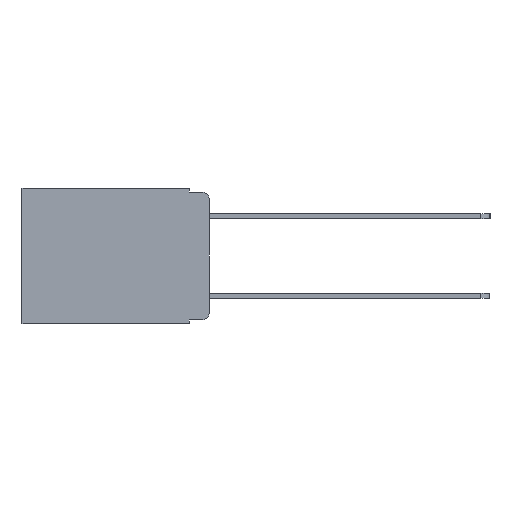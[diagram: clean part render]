
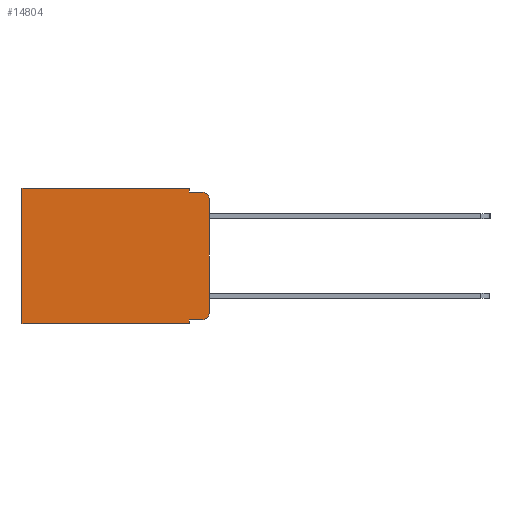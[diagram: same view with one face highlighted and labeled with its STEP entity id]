
A CAD part, left-side view. The second image highlights one B-rep face of the part: STEP entity #14804.
In plain terms, the highlighted planar face has unit normal (-1, 0, 0).
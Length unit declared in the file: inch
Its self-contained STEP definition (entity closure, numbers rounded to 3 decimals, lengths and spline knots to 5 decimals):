
#355 = CARTESIAN_POINT ( 'NONE',  ( 0.298, 0.02, -0.03 ) ) ;
#734 = ORIENTED_EDGE ( 'NONE', *, *, #15490, .T. ) ;
#1044 = DIRECTION ( 'NONE',  ( -1., 0., 0. ) ) ;
#1151 = CARTESIAN_POINT ( 'NONE',  ( 0.298, 0., 0. ) ) ;
#1169 = EDGE_CURVE ( 'NONE', #6300, #10771, #10033, .T. ) ;
#1171 = CARTESIAN_POINT ( 'NONE',  ( 0.298, 0.051, 0. ) ) ;
#1495 = VERTEX_POINT ( 'NONE', #5704 ) ;
#1880 = DIRECTION ( 'NONE',  ( 0., 0., -1. ) ) ;
#1925 = EDGE_LOOP ( 'NONE', ( #15709, #5571, #3028, #11888, #15908, #13172, #9977, #6684, #4193, #734 ) ) ;
#2404 = VECTOR ( 'NONE', #9166, 39.37008 ) ;
#2518 = CARTESIAN_POINT ( 'NONE',  ( 0.298, 0., -0.03 ) ) ;
#2577 = VECTOR ( 'NONE', #15664, 39.37008 ) ;
#2625 = DIRECTION ( 'NONE',  ( 0., 0., -1. ) ) ;
#3028 = ORIENTED_EDGE ( 'NONE', *, *, #18139, .F. ) ;
#3727 = CARTESIAN_POINT ( 'NONE',  ( 0.298, 0., -0.343 ) ) ;
#3985 = CARTESIAN_POINT ( 'NONE',  ( 0.298, 0.051, -0.333 ) ) ;
#4073 = LINE ( 'NONE', #1151, #11562 ) ;
#4193 = ORIENTED_EDGE ( 'NONE', *, *, #10591, .T. ) ;
#4564 = CIRCLE ( 'NONE', #8751, 0.02 ) ;
#4751 = DIRECTION ( 'NONE',  ( 0., -1., 0. ) ) ;
#5084 = VERTEX_POINT ( 'NONE', #9344 ) ;
#5256 = PLANE ( 'NONE',  #6609 ) ;
#5445 = CARTESIAN_POINT ( 'NONE',  ( 0.298, 0.02, -0.333 ) ) ;
#5571 = ORIENTED_EDGE ( 'NONE', *, *, #13272, .T. ) ;
#5581 = CARTESIAN_POINT ( 'NONE',  ( 0.298, 0., 0. ) ) ;
#5704 = CARTESIAN_POINT ( 'NONE',  ( 0.298, 0.051, -0.343 ) ) ;
#6225 = CIRCLE ( 'NONE', #15135, 0.02 ) ;
#6254 = VERTEX_POINT ( 'NONE', #2518 ) ;
#6300 = VERTEX_POINT ( 'NONE', #1171 ) ;
#6370 = EDGE_CURVE ( 'NONE', #6946, #1495, #15017, .T. ) ;
#6609 = AXIS2_PLACEMENT_3D ( 'NONE', #8135, #17629, #9533 ) ;
#6635 = DIRECTION ( 'NONE',  ( 0., 1., 0. ) ) ;
#6684 = ORIENTED_EDGE ( 'NONE', *, *, #6370, .F. ) ;
#6946 = VERTEX_POINT ( 'NONE', #3985 ) ;
#6956 = EDGE_CURVE ( 'NONE', #10771, #8668, #11997, .T. ) ;
#6974 = EDGE_CURVE ( 'NONE', #6254, #5084, #4073, .T. ) ;
#7636 = VERTEX_POINT ( 'NONE', #5445 ) ;
#8066 = VECTOR ( 'NONE', #4751, 39.37008 ) ;
#8135 = CARTESIAN_POINT ( 'NONE',  ( 0.298, 0., 0. ) ) ;
#8584 = CARTESIAN_POINT ( 'NONE',  ( 0.298, 0.051, 0. ) ) ;
#8668 = VERTEX_POINT ( 'NONE', #14186 ) ;
#8751 = AXIS2_PLACEMENT_3D ( 'NONE', #9694, #1044, #11049 ) ;
#8850 = DIRECTION ( 'NONE',  ( 0., 0., -1. ) ) ;
#9098 = VECTOR ( 'NONE', #8850, 39.37008 ) ;
#9166 = DIRECTION ( 'NONE',  ( 0., 1., 0. ) ) ;
#9230 = VERTEX_POINT ( 'NONE', #11416 ) ;
#9344 = CARTESIAN_POINT ( 'NONE',  ( 0.298, 0., -0.313 ) ) ;
#9533 = DIRECTION ( 'NONE',  ( 0., 0., -1. ) ) ;
#9694 = CARTESIAN_POINT ( 'NONE',  ( 0.298, 0.02, -0.313 ) ) ;
#9735 = DIRECTION ( 'NONE',  ( 0., 0., -1. ) ) ;
#9973 = DIRECTION ( 'NONE',  ( 0., 0., -1. ) ) ;
#9977 = ORIENTED_EDGE ( 'NONE', *, *, #14113, .F. ) ;
#10016 = CARTESIAN_POINT ( 'NONE',  ( 0.298, 0.02, -0.01 ) ) ;
#10033 = LINE ( 'NONE', #5581, #2404 ) ;
#10454 = DIRECTION ( 'NONE',  ( -1., 0., 0. ) ) ;
#10591 = EDGE_CURVE ( 'NONE', #6946, #7636, #16122, .T. ) ;
#10771 = VERTEX_POINT ( 'NONE', #15990 ) ;
#11049 = DIRECTION ( 'NONE',  ( 0., 0., -1. ) ) ;
#11215 = EDGE_CURVE ( 'NONE', #6300, #9230, #17580, .T. ) ;
#11416 = CARTESIAN_POINT ( 'NONE',  ( 0.298, 0.051, -0.01 ) ) ;
#11562 = VECTOR ( 'NONE', #2625, 39.37008 ) ;
#11888 = ORIENTED_EDGE ( 'NONE', *, *, #11215, .F. ) ;
#11997 = LINE ( 'NONE', #13815, #12417 ) ;
#12052 = VERTEX_POINT ( 'NONE', #10016 ) ;
#12417 = VECTOR ( 'NONE', #9735, 39.37008 ) ;
#12443 = FACE_OUTER_BOUND ( 'NONE', #1925, .T. ) ;
#13117 = CARTESIAN_POINT ( 'NONE',  ( 0.298, 0.051, -0.01 ) ) ;
#13172 = ORIENTED_EDGE ( 'NONE', *, *, #6956, .T. ) ;
#13272 = EDGE_CURVE ( 'NONE', #6254, #12052, #6225, .T. ) ;
#13815 = CARTESIAN_POINT ( 'NONE',  ( 0.298, 0.473, 0. ) ) ;
#14113 = EDGE_CURVE ( 'NONE', #1495, #8668, #14418, .T. ) ;
#14186 = CARTESIAN_POINT ( 'NONE',  ( 0.298, 0.473, -0.343 ) ) ;
#14286 = CARTESIAN_POINT ( 'NONE',  ( 0.298, 0.051, 0. ) ) ;
#14306 = CARTESIAN_POINT ( 'NONE',  ( 0.298, 0.051, -0.333 ) ) ;
#14418 = LINE ( 'NONE', #3727, #17547 ) ;
#14804 = ADVANCED_FACE ( 'NONE', ( #12443 ), #5256, .F. ) ;
#15017 = LINE ( 'NONE', #8584, #17292 ) ;
#15135 = AXIS2_PLACEMENT_3D ( 'NONE', #355, #10454, #1880 ) ;
#15328 = LINE ( 'NONE', #13117, #8066 ) ;
#15490 = EDGE_CURVE ( 'NONE', #7636, #5084, #4564, .T. ) ;
#15664 = DIRECTION ( 'NONE',  ( 0., -1., 0. ) ) ;
#15709 = ORIENTED_EDGE ( 'NONE', *, *, #6974, .F. ) ;
#15908 = ORIENTED_EDGE ( 'NONE', *, *, #1169, .T. ) ;
#15990 = CARTESIAN_POINT ( 'NONE',  ( 0.298, 0.473, 0. ) ) ;
#16122 = LINE ( 'NONE', #14306, #2577 ) ;
#17292 = VECTOR ( 'NONE', #9973, 39.37008 ) ;
#17547 = VECTOR ( 'NONE', #6635, 39.37008 ) ;
#17580 = LINE ( 'NONE', #14286, #9098 ) ;
#17629 = DIRECTION ( 'NONE',  ( 1., 0., 0. ) ) ;
#18139 = EDGE_CURVE ( 'NONE', #9230, #12052, #15328, .T. ) ;
